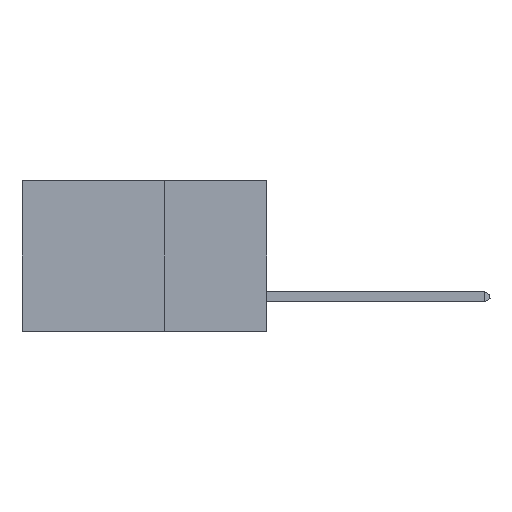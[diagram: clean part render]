
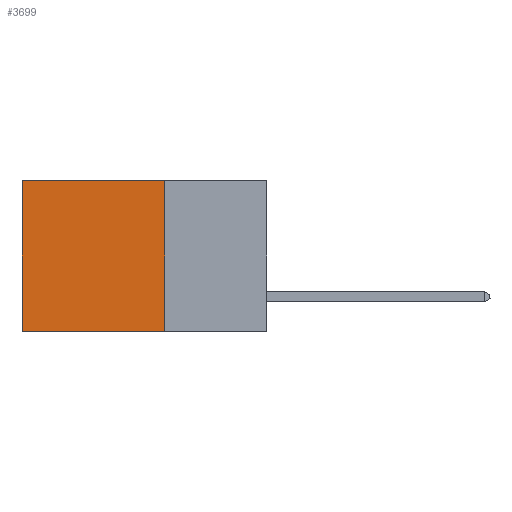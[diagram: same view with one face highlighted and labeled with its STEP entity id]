
A CAD part, left-side view. The second image highlights one B-rep face of the part: STEP entity #3699.
In plain terms, the highlighted planar face has unit normal (-1, 0, 0).
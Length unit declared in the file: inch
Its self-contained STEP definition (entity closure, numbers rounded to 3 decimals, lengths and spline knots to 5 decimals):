
#1996 = LINE ( 'NONE', #45754, #28330 ) ;
#2126 = PLANE ( 'NONE',  #12278 ) ;
#3699 = ADVANCED_FACE ( 'NONE', ( #7612 ), #2126, .F. ) ;
#7612 = FACE_OUTER_BOUND ( 'NONE', #42573, .T. ) ;
#11010 = ORIENTED_EDGE ( 'NONE', *, *, #25487, .T. ) ;
#11294 = LINE ( 'NONE', #11852, #23645 ) ;
#11852 = CARTESIAN_POINT ( 'NONE',  ( 0.2875, 0.25, -0.37 ) ) ;
#12278 = AXIS2_PLACEMENT_3D ( 'NONE', #42496, #44015, #43310 ) ;
#12573 = ORIENTED_EDGE ( 'NONE', *, *, #24977, .T. ) ;
#12707 = CARTESIAN_POINT ( 'NONE',  ( 0.2875, 0.25, 0. ) ) ;
#13690 = VECTOR ( 'NONE', #38283, 39.37008 ) ;
#14769 = LINE ( 'NONE', #42020, #13690 ) ;
#14963 = DIRECTION ( 'NONE',  ( 0., 0., -1. ) ) ;
#15254 = LINE ( 'NONE', #36545, #20378 ) ;
#16214 = CARTESIAN_POINT ( 'NONE',  ( 0.2875, 0.6, -0.37 ) ) ;
#20378 = VECTOR ( 'NONE', #14963, 39.37008 ) ;
#22511 = DIRECTION ( 'NONE',  ( 0., 1., 0. ) ) ;
#22750 = CARTESIAN_POINT ( 'NONE',  ( 0.2875, 0.25, -0.37 ) ) ;
#23645 = VECTOR ( 'NONE', #22511, 39.37008 ) ;
#23694 = VERTEX_POINT ( 'NONE', #12707 ) ;
#24977 = EDGE_CURVE ( 'NONE', #23694, #39461, #14769, .T. ) ;
#25487 = EDGE_CURVE ( 'NONE', #39461, #45925, #15254, .T. ) ;
#28330 = VECTOR ( 'NONE', #37494, 39.37008 ) ;
#30333 = EDGE_CURVE ( 'NONE', #23694, #35561, #1996, .T. ) ;
#35561 = VERTEX_POINT ( 'NONE', #22750 ) ;
#36545 = CARTESIAN_POINT ( 'NONE',  ( 0.2875, 0.6, 0. ) ) ;
#37494 = DIRECTION ( 'NONE',  ( 0., 0., -1. ) ) ;
#37558 = ORIENTED_EDGE ( 'NONE', *, *, #30333, .F. ) ;
#38283 = DIRECTION ( 'NONE',  ( 0., 1., 0. ) ) ;
#39461 = VERTEX_POINT ( 'NONE', #40353 ) ;
#39746 = ORIENTED_EDGE ( 'NONE', *, *, #41534, .F. ) ;
#40353 = CARTESIAN_POINT ( 'NONE',  ( 0.2875, 0.6, 0. ) ) ;
#41534 = EDGE_CURVE ( 'NONE', #35561, #45925, #11294, .T. ) ;
#42020 = CARTESIAN_POINT ( 'NONE',  ( 0.2875, 0.25, 0. ) ) ;
#42496 = CARTESIAN_POINT ( 'NONE',  ( 0.2875, 0.25, 0. ) ) ;
#42573 = EDGE_LOOP ( 'NONE', ( #11010, #39746, #37558, #12573 ) ) ;
#43310 = DIRECTION ( 'NONE',  ( 0., 0., -1. ) ) ;
#44015 = DIRECTION ( 'NONE',  ( 1., 0., 0. ) ) ;
#45754 = CARTESIAN_POINT ( 'NONE',  ( 0.2875, 0.25, 0. ) ) ;
#45925 = VERTEX_POINT ( 'NONE', #16214 ) ;
